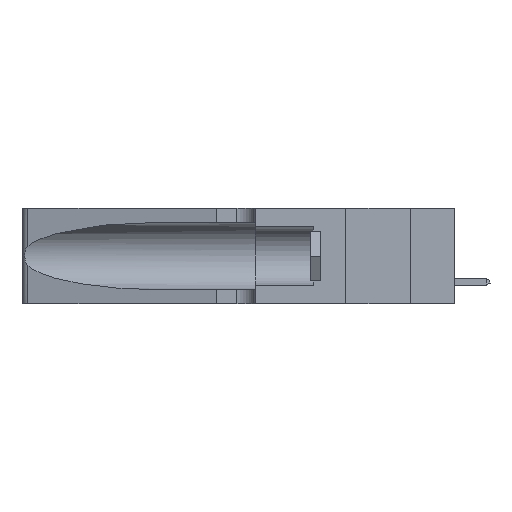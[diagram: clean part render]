
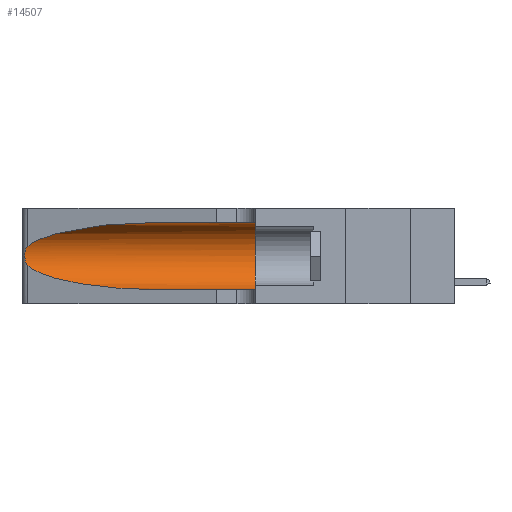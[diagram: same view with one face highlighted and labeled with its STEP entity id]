
A CAD part, left-side view. The second image highlights one B-rep face of the part: STEP entity #14507.
In plain terms, the highlighted cylindrical face has radius 3.308 mm (diameter 6.617 mm), a partial arc.
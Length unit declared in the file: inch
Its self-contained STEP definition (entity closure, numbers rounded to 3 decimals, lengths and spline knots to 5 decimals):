
#1227 = VECTOR ( 'NONE', #22388, 39.37008 ) ;
#1247 = CARTESIAN_POINT ( 'NONE',  ( 0.26018, 1.23835, 0.19895 ) ) ;
#2474 =( BOUNDED_CURVE ( )  B_SPLINE_CURVE ( 3, ( #7991, #33799, #31548, #10644 ),
 .UNSPECIFIED., .F., .T. ) 
 B_SPLINE_CURVE_WITH_KNOTS ( ( 4, 4 ),
 ( 1.5708, 2.84003 ),
 .UNSPECIFIED. ) 
 CURVE ( )  GEOMETRIC_REPRESENTATION_ITEM ( )  RATIONAL_B_SPLINE_CURVE ( ( 1., 0.87, 0.87, 1. ) ) 
 REPRESENTATION_ITEM ( '' )  );
#4528 = LINE ( 'NONE', #26553, #30837 ) ;
#5891 = CARTESIAN_POINT ( 'NONE',  ( 0.1305, 1.61858, 0.185 ) ) ;
#6552 = CARTESIAN_POINT ( 'NONE',  ( 0.18966, 0.96281, 0.05475 ) ) ;
#6632 = DIRECTION ( 'NONE',  ( 0., 0., 1. ) ) ;
#6721 = CARTESIAN_POINT ( 'NONE',  ( 0.26017, 1.23833, 0.17102 ) ) ;
#7195 = CARTESIAN_POINT ( 'NONE',  ( 0.1305, 0.35, 0.05475 ) ) ;
#7664 =( BOUNDED_CURVE ( )  B_SPLINE_CURVE ( 3, ( #14551, #9619, #6552, #32811 ),
 .UNSPECIFIED., .F., .T. ) 
 B_SPLINE_CURVE_WITH_KNOTS ( ( 4, 4 ),
 ( 3.44316, 4.71239 ),
 .UNSPECIFIED. ) 
 CURVE ( )  GEOMETRIC_REPRESENTATION_ITEM ( )  RATIONAL_B_SPLINE_CURVE ( ( 1., 0.87, 0.87, 1. ) ) 
 REPRESENTATION_ITEM ( '' )  );
#7991 = CARTESIAN_POINT ( 'NONE',  ( 0.1305, 0.72297, 0.31525 ) ) ;
#8552 = CARTESIAN_POINT ( 'NONE',  ( 0.25487, 1.22718, 0.22369 ) ) ;
#8895 = CARTESIAN_POINT ( 'NONE',  ( 0.25487, 1.22718, 0.14631 ) ) ;
#9523 = CYLINDRICAL_SURFACE ( 'NONE', #25783, 0.13025 ) ;
#9619 = CARTESIAN_POINT ( 'NONE',  ( 0.2373, 1.15595, 0.08982 ) ) ;
#10644 = CARTESIAN_POINT ( 'NONE',  ( 0.25487, 1.22718, 0.22369 ) ) ;
#10716 = DIRECTION ( 'NONE',  ( 0., -1., 0. ) ) ;
#11306 = CARTESIAN_POINT ( 'NONE',  ( 0.25555, 1.22994, 0.2215 ) ) ;
#11795 = VERTEX_POINT ( 'NONE', #26919 ) ;
#13664 = EDGE_CURVE ( 'NONE', #11795, #25333, #7664, .T. ) ;
#13879 = EDGE_CURVE ( 'NONE', #28477, #29547, #2474, .T. ) ;
#14234 = CARTESIAN_POINT ( 'NONE',  ( 0.1305, 1.61858, 0.05475 ) ) ;
#14410 = VERTEX_POINT ( 'NONE', #20656 ) ;
#14495 = CARTESIAN_POINT ( 'NONE',  ( 0.26075, 1.23896, 0.178 ) ) ;
#14507 = ADVANCED_FACE ( 'NONE', ( #27604 ), #9523, .F. ) ;
#14551 = CARTESIAN_POINT ( 'NONE',  ( 0.25487, 1.22718, 0.14631 ) ) ;
#14624 = CARTESIAN_POINT ( 'NONE',  ( 0.25639, 1.23184, 0.21858 ) ) ;
#14642 = DIRECTION ( 'NONE',  ( 0., 1., 0. ) ) ;
#15159 = LINE ( 'NONE', #14234, #1227 ) ;
#15361 = ORIENTED_EDGE ( 'NONE', *, *, #24851, .F. ) ;
#15523 = ORIENTED_EDGE ( 'NONE', *, *, #13664, .T. ) ;
#15594 = EDGE_LOOP ( 'NONE', ( #28374, #29772, #15523, #27395, #32664, #15361 ) ) ;
#17177 = CARTESIAN_POINT ( 'NONE',  ( 0.1305, 0.35, 0.185 ) ) ;
#17230 = CIRCLE ( 'NONE', #33527, 0.13025 ) ;
#20656 = CARTESIAN_POINT ( 'NONE',  ( 0.1305, 0.35, 0.31525 ) ) ;
#22191 = CARTESIAN_POINT ( 'NONE',  ( 0.26075, 1.23896, 0.19203 ) ) ;
#22388 = DIRECTION ( 'NONE',  ( 0., -1., 0. ) ) ;
#24249 = DIRECTION ( 'NONE',  ( 0., -1., 0. ) ) ;
#24625 = CARTESIAN_POINT ( 'NONE',  ( 0.25856, 1.23593, 0.16098 ) ) ;
#24851 = EDGE_CURVE ( 'NONE', #28477, #14410, #4528, .T. ) ;
#24852 = CARTESIAN_POINT ( 'NONE',  ( 0.25789, 1.23486, 0.15765 ) ) ;
#25193 = VERTEX_POINT ( 'NONE', #7195 ) ;
#25333 = VERTEX_POINT ( 'NONE', #25992 ) ;
#25459 = EDGE_CURVE ( 'NONE', #25333, #25193, #15159, .T. ) ;
#25783 = AXIS2_PLACEMENT_3D ( 'NONE', #5891, #24249, #32179 ) ;
#25977 = CARTESIAN_POINT ( 'NONE',  ( 0.1305, 0.72297, 0.31525 ) ) ;
#25992 = CARTESIAN_POINT ( 'NONE',  ( 0.1305, 0.72297, 0.05475 ) ) ;
#26553 = CARTESIAN_POINT ( 'NONE',  ( 0.1305, 1.61858, 0.31525 ) ) ;
#26919 = CARTESIAN_POINT ( 'NONE',  ( 0.25487, 1.22718, 0.14631 ) ) ;
#27395 = ORIENTED_EDGE ( 'NONE', *, *, #25459, .T. ) ;
#27604 = FACE_OUTER_BOUND ( 'NONE', #15594, .T. ) ;
#28374 = ORIENTED_EDGE ( 'NONE', *, *, #13879, .T. ) ;
#28477 = VERTEX_POINT ( 'NONE', #25977 ) ;
#29375 = EDGE_CURVE ( 'NONE', #14410, #25193, #17230, .T. ) ;
#29547 = VERTEX_POINT ( 'NONE', #33771 ) ;
#29575 = B_SPLINE_CURVE_WITH_KNOTS ( 'NONE', 3,
 ( #8552, #11306, #14624, #29919, #30271, #1247, #22191, #14495, #6721, #24625, #24852, #32868, #30145, #8895 ),
 .UNSPECIFIED., .F., .F.,
 ( 4, 2, 2, 2, 2, 2, 4 ),
 ( 0., 0.00027, 0.00053, 0.00107, 0.0016, 0.00187, 0.00214 ),
 .UNSPECIFIED. ) ;
#29772 = ORIENTED_EDGE ( 'NONE', *, *, #33036, .T. ) ;
#29919 = CARTESIAN_POINT ( 'NONE',  ( 0.25787, 1.23484, 0.2124 ) ) ;
#30145 = CARTESIAN_POINT ( 'NONE',  ( 0.25555, 1.22993, 0.14849 ) ) ;
#30271 = CARTESIAN_POINT ( 'NONE',  ( 0.25854, 1.2359, 0.20912 ) ) ;
#30837 = VECTOR ( 'NONE', #10716, 39.37008 ) ;
#31548 = CARTESIAN_POINT ( 'NONE',  ( 0.2373, 1.15595, 0.28018 ) ) ;
#32179 = DIRECTION ( 'NONE',  ( 0., 0., -1. ) ) ;
#32664 = ORIENTED_EDGE ( 'NONE', *, *, #29375, .F. ) ;
#32811 = CARTESIAN_POINT ( 'NONE',  ( 0.1305, 0.72297, 0.05475 ) ) ;
#32868 = CARTESIAN_POINT ( 'NONE',  ( 0.25639, 1.23186, 0.15144 ) ) ;
#33036 = EDGE_CURVE ( 'NONE', #29547, #11795, #29575, .T. ) ;
#33527 = AXIS2_PLACEMENT_3D ( 'NONE', #17177, #14642, #6632 ) ;
#33771 = CARTESIAN_POINT ( 'NONE',  ( 0.25487, 1.22718, 0.22369 ) ) ;
#33799 = CARTESIAN_POINT ( 'NONE',  ( 0.18966, 0.96281, 0.31525 ) ) ;
